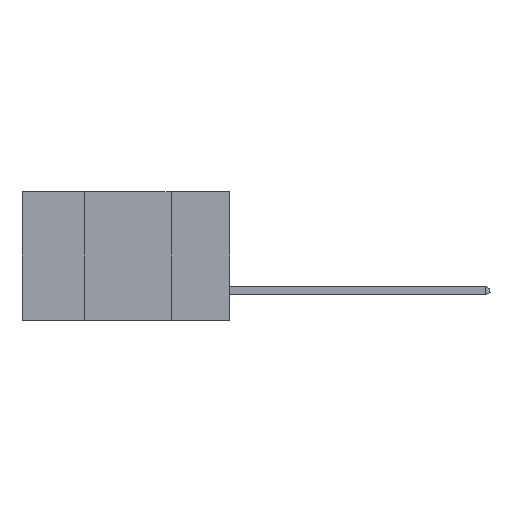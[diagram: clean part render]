
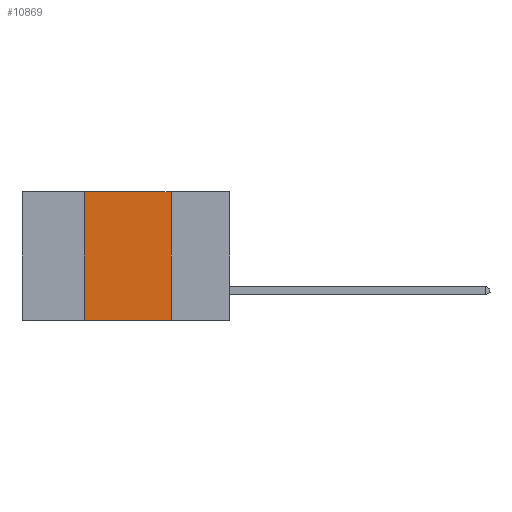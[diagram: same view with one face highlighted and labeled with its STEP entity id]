
A CAD part, left-side view. The second image highlights one B-rep face of the part: STEP entity #10869.
In plain terms, the highlighted planar face has unit normal (-1, 0, 0).
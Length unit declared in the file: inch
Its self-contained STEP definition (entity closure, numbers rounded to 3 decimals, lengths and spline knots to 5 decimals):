
#926 = ORIENTED_EDGE ( 'NONE', *, *, #9976, .T. ) ;
#1226 = VECTOR ( 'NONE', #9767, 39.37008 ) ;
#1468 = EDGE_CURVE ( 'NONE', #13948, #6386, #8713, .T. ) ;
#1566 = VECTOR ( 'NONE', #7546, 39.37008 ) ;
#1745 = ORIENTED_EDGE ( 'NONE', *, *, #11783, .F. ) ;
#2338 = EDGE_CURVE ( 'NONE', #10276, #13948, #6908, .T. ) ;
#2667 = CARTESIAN_POINT ( 'NONE',  ( 0., 0.42, 0. ) ) ;
#3569 = CARTESIAN_POINT ( 'NONE',  ( 0., 0.17, -0.37 ) ) ;
#3738 = LINE ( 'NONE', #6604, #9084 ) ;
#4310 = DIRECTION ( 'NONE',  ( 1., 0., 0. ) ) ;
#4462 = CARTESIAN_POINT ( 'NONE',  ( 0., 0.6, 0. ) ) ;
#6386 = VERTEX_POINT ( 'NONE', #12721 ) ;
#6604 = CARTESIAN_POINT ( 'NONE',  ( 0., 0.6, -0.37 ) ) ;
#6751 = DIRECTION ( 'NONE',  ( 0., -1., 0. ) ) ;
#6908 = LINE ( 'NONE', #13119, #1566 ) ;
#6919 = AXIS2_PLACEMENT_3D ( 'NONE', #4462, #4310, #13695 ) ;
#7181 = DIRECTION ( 'NONE',  ( 0., 0., -1. ) ) ;
#7546 = DIRECTION ( 'NONE',  ( 0., 0., 1. ) ) ;
#8356 = FACE_OUTER_BOUND ( 'NONE', #13208, .T. ) ;
#8713 = LINE ( 'NONE', #14311, #1226 ) ;
#9084 = VECTOR ( 'NONE', #6751, 39.37008 ) ;
#9328 = VERTEX_POINT ( 'NONE', #3569 ) ;
#9767 = DIRECTION ( 'NONE',  ( 0., -1., 0. ) ) ;
#9976 = EDGE_CURVE ( 'NONE', #10276, #9328, #3738, .T. ) ;
#10276 = VERTEX_POINT ( 'NONE', #10443 ) ;
#10443 = CARTESIAN_POINT ( 'NONE',  ( 0., 0.42, -0.37 ) ) ;
#10869 = ADVANCED_FACE ( 'NONE', ( #8356 ), #11291, .F. ) ;
#11291 = PLANE ( 'NONE',  #6919 ) ;
#11501 = VECTOR ( 'NONE', #7181, 39.37008 ) ;
#11783 = EDGE_CURVE ( 'NONE', #6386, #9328, #11861, .T. ) ;
#11787 = ORIENTED_EDGE ( 'NONE', *, *, #1468, .F. ) ;
#11861 = LINE ( 'NONE', #14001, #11501 ) ;
#12721 = CARTESIAN_POINT ( 'NONE',  ( 0., 0.17, 0. ) ) ;
#13118 = ORIENTED_EDGE ( 'NONE', *, *, #2338, .F. ) ;
#13119 = CARTESIAN_POINT ( 'NONE',  ( 0., 0.42, 0. ) ) ;
#13208 = EDGE_LOOP ( 'NONE', ( #1745, #11787, #13118, #926 ) ) ;
#13695 = DIRECTION ( 'NONE',  ( 0., 0., -1. ) ) ;
#13948 = VERTEX_POINT ( 'NONE', #2667 ) ;
#14001 = CARTESIAN_POINT ( 'NONE',  ( 0., 0.17, 0. ) ) ;
#14311 = CARTESIAN_POINT ( 'NONE',  ( 0., 0.6, 0. ) ) ;
